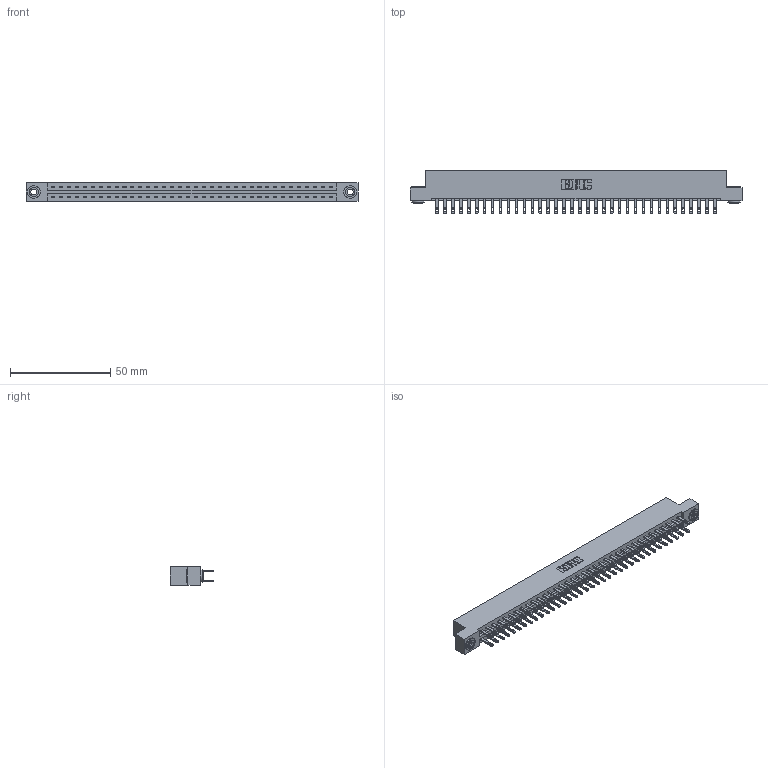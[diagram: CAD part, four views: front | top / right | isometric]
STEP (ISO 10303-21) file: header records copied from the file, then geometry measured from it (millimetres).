
FILE_DESCRIPTION (( 'STEP AP203' ), '1' );
FILE_NAME ('337-072-500-203.STEP', '2018-08-11T13:40:45', ( '' ), ( '' ), 'SwSTEP 2.0', 'SolidWorks 2016', '' );
FILE_SCHEMA (( 'CONFIG_CONTROL_DESIGN' ));
Length unit declared in the file: inch
Products named in the file (4): 337 Part_Flush Mounting Lugs - 0.156 Dia-TH; 345-292-001_345-293-100; 345-250-002_345-250-002-102; 337-072-500-203
Assembly tree (75 placements, depth 2):
  337-072-500-203
    337 Part_Flush Mounting Lugs - 0.156 Dia-TH
    345-292-001_345-293-100  x72
    345-250-002_345-250-002-102  x2
Bounding box: 165.66 x 21.85 x 9.4 mm (x, y, z)
Volume: 17618 mm3; surface area: 20882.2 mm2
Topology: 75 solids, 75 shells, 3752 faces, 11403 edges, 7598 vertices
Faces by surface type: plane 2384, cylinder 1360, cone 8
Entity records: 29268 total; most frequent: CARTESIAN_POINT 4909, ORIENTED_EDGE 4838, DIRECTION 4221, EDGE_CURVE 2419, VECTOR 2263, LINE 2263, VERTEX_POINT 1610, AXIS2_PLACEMENT_3D 979
